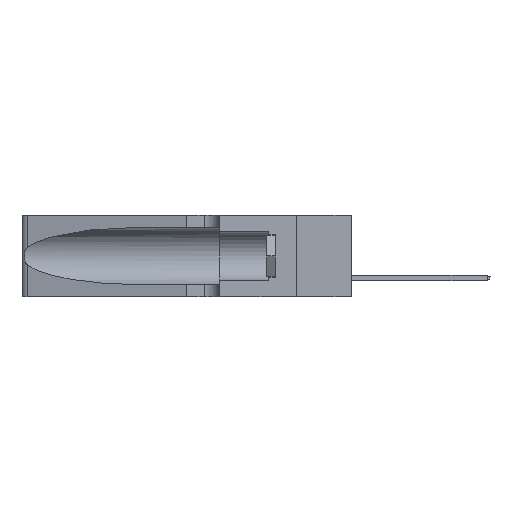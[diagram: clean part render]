
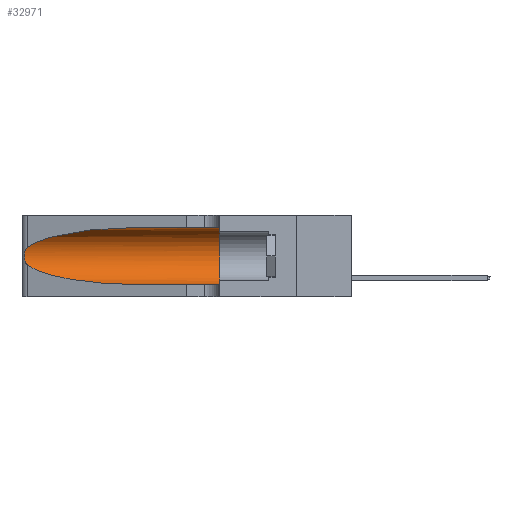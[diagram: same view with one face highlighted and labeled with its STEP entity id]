
A CAD part, left-side view. The second image highlights one B-rep face of the part: STEP entity #32971.
In plain terms, the highlighted cylindrical face has radius 3.308 mm (diameter 6.617 mm), a partial arc.
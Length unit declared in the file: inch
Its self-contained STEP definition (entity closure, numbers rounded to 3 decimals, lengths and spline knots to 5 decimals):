
#590 = B_SPLINE_CURVE_WITH_KNOTS ( 'NONE', 3,
 ( #28470, #6523, #12663, #15526, #28222, #18854, #6634, #32291, #28860, #32018, #3643, #35462, #25619, #20084 ),
 .UNSPECIFIED., .F., .F.,
 ( 4, 2, 2, 2, 2, 2, 4 ),
 ( 0., 0.00027, 0.00053, 0.00107, 0.0016, 0.00187, 0.00214 ),
 .UNSPECIFIED. ) ;
#1270 = EDGE_CURVE ( 'NONE', #7124, #5711, #590, .T. ) ;
#3038 = AXIS2_PLACEMENT_3D ( 'NONE', #21301, #14774, #14363 ) ;
#3049 = ORIENTED_EDGE ( 'NONE', *, *, #1270, .T. ) ;
#3282 = DIRECTION ( 'NONE',  ( 0., 0., 1. ) ) ;
#3581 = VECTOR ( 'NONE', #18089, 39.37008 ) ;
#3643 = CARTESIAN_POINT ( 'NONE',  ( 0.25789, 1.23486, 0.15765 ) ) ;
#5711 = VERTEX_POINT ( 'NONE', #28642 ) ;
#6042 = LINE ( 'NONE', #11908, #3581 ) ;
#6436 = EDGE_CURVE ( 'NONE', #27913, #34829, #6042, .T. ) ;
#6523 = CARTESIAN_POINT ( 'NONE',  ( 0.25555, 1.22994, 0.2215 ) ) ;
#6594 = EDGE_CURVE ( 'NONE', #19591, #29573, #38397, .T. ) ;
#6634 = CARTESIAN_POINT ( 'NONE',  ( 0.26075, 1.23896, 0.19203 ) ) ;
#6977 = CARTESIAN_POINT ( 'NONE',  ( 0.2373, 1.15595, 0.28018 ) ) ;
#7124 = VERTEX_POINT ( 'NONE', #30525 ) ;
#7624 = ORIENTED_EDGE ( 'NONE', *, *, #20882, .F. ) ;
#10543 = CARTESIAN_POINT ( 'NONE',  ( 0.1305, 0.72297, 0.31525 ) ) ;
#11908 = CARTESIAN_POINT ( 'NONE',  ( 0.1305, 1.61858, 0.31525 ) ) ;
#12589 = CARTESIAN_POINT ( 'NONE',  ( 0.1305, 0.72297, 0.05475 ) ) ;
#12663 = CARTESIAN_POINT ( 'NONE',  ( 0.25639, 1.23184, 0.21858 ) ) ;
#13790 = CARTESIAN_POINT ( 'NONE',  ( 0.1305, 1.61858, 0.05475 ) ) ;
#14363 = DIRECTION ( 'NONE',  ( 0., 0., -1. ) ) ;
#14774 = DIRECTION ( 'NONE',  ( 0., -1., 0. ) ) ;
#15526 = CARTESIAN_POINT ( 'NONE',  ( 0.25787, 1.23484, 0.2124 ) ) ;
#15760 = EDGE_CURVE ( 'NONE', #5711, #19591, #19401, .T. ) ;
#15910 = CARTESIAN_POINT ( 'NONE',  ( 0.2373, 1.15595, 0.08982 ) ) ;
#16202 = CARTESIAN_POINT ( 'NONE',  ( 0.25487, 1.22718, 0.14631 ) ) ;
#18089 = DIRECTION ( 'NONE',  ( 0., -1., 0. ) ) ;
#18190 = CARTESIAN_POINT ( 'NONE',  ( 0.1305, 0.35, 0.05475 ) ) ;
#18854 = CARTESIAN_POINT ( 'NONE',  ( 0.26018, 1.23835, 0.19895 ) ) ;
#19401 =( BOUNDED_CURVE ( )  B_SPLINE_CURVE ( 3, ( #16202, #15910, #22053, #25742 ),
 .UNSPECIFIED., .F., .T. ) 
 B_SPLINE_CURVE_WITH_KNOTS ( ( 4, 4 ),
 ( 3.44316, 4.71239 ),
 .UNSPECIFIED. ) 
 CURVE ( )  GEOMETRIC_REPRESENTATION_ITEM ( )  RATIONAL_B_SPLINE_CURVE ( ( 1., 0.87, 0.87, 1. ) ) 
 REPRESENTATION_ITEM ( '' )  );
#19591 = VERTEX_POINT ( 'NONE', #12589 ) ;
#20084 = CARTESIAN_POINT ( 'NONE',  ( 0.25487, 1.22718, 0.14631 ) ) ;
#20882 = EDGE_CURVE ( 'NONE', #34829, #29573, #32605, .T. ) ;
#21301 = CARTESIAN_POINT ( 'NONE',  ( 0.1305, 1.61858, 0.185 ) ) ;
#21989 =( BOUNDED_CURVE ( )  B_SPLINE_CURVE ( 3, ( #10543, #38695, #6977, #32099 ),
 .UNSPECIFIED., .F., .F. ) 
 B_SPLINE_CURVE_WITH_KNOTS ( ( 4, 4 ),
 ( 1.5708, 2.84003 ),
 .UNSPECIFIED. ) 
 CURVE ( )  GEOMETRIC_REPRESENTATION_ITEM ( )  RATIONAL_B_SPLINE_CURVE ( ( 1., 0.87, 0.87, 1. ) ) 
 REPRESENTATION_ITEM ( '' )  );
#22053 = CARTESIAN_POINT ( 'NONE',  ( 0.18966, 0.96281, 0.05475 ) ) ;
#22967 = ORIENTED_EDGE ( 'NONE', *, *, #6594, .T. ) ;
#24480 = EDGE_LOOP ( 'NONE', ( #25202, #3049, #33917, #22967, #7624, #35299 ) ) ;
#25202 = ORIENTED_EDGE ( 'NONE', *, *, #35817, .T. ) ;
#25619 = CARTESIAN_POINT ( 'NONE',  ( 0.25555, 1.22993, 0.14849 ) ) ;
#25742 = CARTESIAN_POINT ( 'NONE',  ( 0.1305, 0.72297, 0.05475 ) ) ;
#26786 = CARTESIAN_POINT ( 'NONE',  ( 0.1305, 0.72297, 0.31525 ) ) ;
#27913 = VERTEX_POINT ( 'NONE', #26786 ) ;
#28222 = CARTESIAN_POINT ( 'NONE',  ( 0.25854, 1.2359, 0.20912 ) ) ;
#28470 = CARTESIAN_POINT ( 'NONE',  ( 0.25487, 1.22718, 0.22369 ) ) ;
#28642 = CARTESIAN_POINT ( 'NONE',  ( 0.25487, 1.22718, 0.14631 ) ) ;
#28679 = AXIS2_PLACEMENT_3D ( 'NONE', #30716, #37172, #3282 ) ;
#28860 = CARTESIAN_POINT ( 'NONE',  ( 0.26017, 1.23833, 0.17102 ) ) ;
#29573 = VERTEX_POINT ( 'NONE', #18190 ) ;
#30525 = CARTESIAN_POINT ( 'NONE',  ( 0.25487, 1.22718, 0.22369 ) ) ;
#30716 = CARTESIAN_POINT ( 'NONE',  ( 0.1305, 0.35, 0.185 ) ) ;
#32018 = CARTESIAN_POINT ( 'NONE',  ( 0.25856, 1.23593, 0.16098 ) ) ;
#32099 = CARTESIAN_POINT ( 'NONE',  ( 0.25487, 1.22718, 0.22369 ) ) ;
#32291 = CARTESIAN_POINT ( 'NONE',  ( 0.26075, 1.23896, 0.178 ) ) ;
#32393 = FACE_OUTER_BOUND ( 'NONE', #24480, .T. ) ;
#32605 = CIRCLE ( 'NONE', #28679, 0.13025 ) ;
#32971 = ADVANCED_FACE ( 'NONE', ( #32393 ), #39328, .F. ) ;
#33917 = ORIENTED_EDGE ( 'NONE', *, *, #15760, .T. ) ;
#34829 = VERTEX_POINT ( 'NONE', #35510 ) ;
#35299 = ORIENTED_EDGE ( 'NONE', *, *, #6436, .F. ) ;
#35462 = CARTESIAN_POINT ( 'NONE',  ( 0.25639, 1.23186, 0.15144 ) ) ;
#35510 = CARTESIAN_POINT ( 'NONE',  ( 0.1305, 0.35, 0.31525 ) ) ;
#35817 = EDGE_CURVE ( 'NONE', #27913, #7124, #21989, .T. ) ;
#36991 = VECTOR ( 'NONE', #39085, 39.37008 ) ;
#37172 = DIRECTION ( 'NONE',  ( 0., 1., 0. ) ) ;
#38397 = LINE ( 'NONE', #13790, #36991 ) ;
#38695 = CARTESIAN_POINT ( 'NONE',  ( 0.18966, 0.96281, 0.31525 ) ) ;
#39085 = DIRECTION ( 'NONE',  ( 0., -1., 0. ) ) ;
#39328 = CYLINDRICAL_SURFACE ( 'NONE', #3038, 0.13025 ) ;
